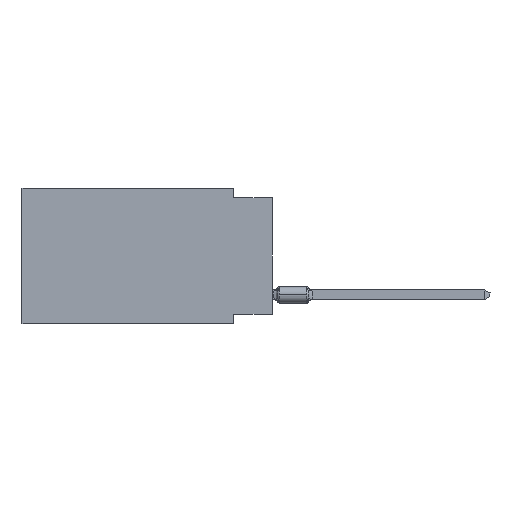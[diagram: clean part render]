
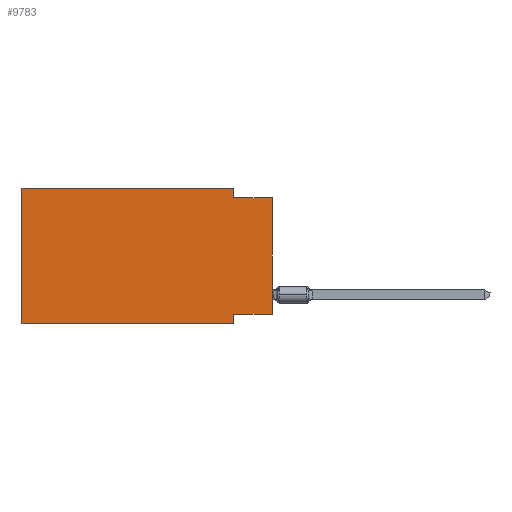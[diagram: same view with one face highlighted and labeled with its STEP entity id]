
A CAD part, left-side view. The second image highlights one B-rep face of the part: STEP entity #9783.
In plain terms, the highlighted planar face has unit normal (-1, 0, 0).
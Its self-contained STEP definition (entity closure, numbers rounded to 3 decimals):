
#138 = VERTEX_POINT ( 'NONE', #35440 ) ;
#205 = CARTESIAN_POINT ( 'NONE',  ( 0., 16.383, 0. ) ) ;
#745 = ORIENTED_EDGE ( 'NONE', *, *, #3948, .F. ) ;
#858 = DIRECTION ( 'NONE',  ( 1., 0., 0. ) ) ;
#873 = LINE ( 'NONE', #11463, #5144 ) ;
#1146 = EDGE_CURVE ( 'NONE', #31662, #40029, #20476, .T. ) ;
#1356 = VERTEX_POINT ( 'NONE', #39842 ) ;
#1871 = VERTEX_POINT ( 'NONE', #23699 ) ;
#2549 = LINE ( 'NONE', #33441, #22198 ) ;
#2625 = CARTESIAN_POINT ( 'NONE',  ( 0., 2.54, -8.89 ) ) ;
#3072 = LINE ( 'NONE', #205, #10060 ) ;
#3726 = FACE_OUTER_BOUND ( 'NONE', #29247, .T. ) ;
#3946 = CARTESIAN_POINT ( 'NONE',  ( 0., 16.383, 0. ) ) ;
#3948 = EDGE_CURVE ( 'NONE', #138, #4525, #3072, .T. ) ;
#4525 = VERTEX_POINT ( 'NONE', #18539 ) ;
#5144 = VECTOR ( 'NONE', #38138, 1000. ) ;
#5912 = LINE ( 'NONE', #2625, #37120 ) ;
#6552 = CARTESIAN_POINT ( 'NONE',  ( 0., 16.383, -8.89 ) ) ;
#6818 = DIRECTION ( 'NONE',  ( 0., 0., -1. ) ) ;
#7232 = VECTOR ( 'NONE', #14367, 1000. ) ;
#7690 = CARTESIAN_POINT ( 'NONE',  ( 0., 0., -8.255 ) ) ;
#9783 = ADVANCED_FACE ( 'NONE', ( #3726 ), #27144, .F. ) ;
#9858 = ORIENTED_EDGE ( 'NONE', *, *, #39372, .T. ) ;
#10060 = VECTOR ( 'NONE', #10582, 1000. ) ;
#10582 = DIRECTION ( 'NONE',  ( 0., 0., 1. ) ) ;
#11132 = CARTESIAN_POINT ( 'NONE',  ( 0., 2.54, -8.89 ) ) ;
#11463 = CARTESIAN_POINT ( 'NONE',  ( 0., 0., 0. ) ) ;
#12871 = DIRECTION ( 'NONE',  ( 0., -1., 0. ) ) ;
#13057 = EDGE_CURVE ( 'NONE', #1871, #35062, #5912, .T. ) ;
#13925 = ORIENTED_EDGE ( 'NONE', *, *, #23157, .F. ) ;
#14367 = DIRECTION ( 'NONE',  ( 0., 1., 0. ) ) ;
#14634 = ORIENTED_EDGE ( 'NONE', *, *, #30219, .F. ) ;
#15038 = DIRECTION ( 'NONE',  ( 0., -1., 0. ) ) ;
#15153 = EDGE_CURVE ( 'NONE', #4525, #31662, #2549, .T. ) ;
#15992 = ORIENTED_EDGE ( 'NONE', *, *, #13057, .F. ) ;
#18539 = CARTESIAN_POINT ( 'NONE',  ( 0., 16.383, 0. ) ) ;
#19082 = VERTEX_POINT ( 'NONE', #7690 ) ;
#20476 = LINE ( 'NONE', #24014, #36927 ) ;
#20486 = DIRECTION ( 'NONE',  ( 0., 0., -1. ) ) ;
#21554 = LINE ( 'NONE', #38530, #35838 ) ;
#22133 = ORIENTED_EDGE ( 'NONE', *, *, #36055, .T. ) ;
#22198 = VECTOR ( 'NONE', #36741, 1000. ) ;
#22958 = VECTOR ( 'NONE', #15038, 1000. ) ;
#23157 = EDGE_CURVE ( 'NONE', #19082, #1871, #36664, .T. ) ;
#23699 = CARTESIAN_POINT ( 'NONE',  ( 0., 2.54, -8.255 ) ) ;
#24014 = CARTESIAN_POINT ( 'NONE',  ( 0., 2.54, 0. ) ) ;
#25016 = ORIENTED_EDGE ( 'NONE', *, *, #15153, .F. ) ;
#26099 = CARTESIAN_POINT ( 'NONE',  ( 0., 0., -8.255 ) ) ;
#26667 = LINE ( 'NONE', #6552, #22958 ) ;
#27144 = PLANE ( 'NONE',  #39819 ) ;
#29247 = EDGE_LOOP ( 'NONE', ( #22133, #14634, #31177, #25016, #745, #9858, #15992, #13925 ) ) ;
#30219 = EDGE_CURVE ( 'NONE', #40029, #1356, #21554, .T. ) ;
#31058 = DIRECTION ( 'NONE',  ( 0., 0., -1. ) ) ;
#31177 = ORIENTED_EDGE ( 'NONE', *, *, #1146, .F. ) ;
#31662 = VERTEX_POINT ( 'NONE', #36081 ) ;
#33441 = CARTESIAN_POINT ( 'NONE',  ( 0., 16.383, 0. ) ) ;
#35062 = VERTEX_POINT ( 'NONE', #11132 ) ;
#35440 = CARTESIAN_POINT ( 'NONE',  ( 0., 16.383, -8.89 ) ) ;
#35838 = VECTOR ( 'NONE', #12871, 1000. ) ;
#36055 = EDGE_CURVE ( 'NONE', #19082, #1356, #873, .T. ) ;
#36081 = CARTESIAN_POINT ( 'NONE',  ( 0., 2.54, 0. ) ) ;
#36664 = LINE ( 'NONE', #26099, #7232 ) ;
#36741 = DIRECTION ( 'NONE',  ( 0., -1., 0. ) ) ;
#36927 = VECTOR ( 'NONE', #31058, 1000. ) ;
#37120 = VECTOR ( 'NONE', #20486, 1000. ) ;
#38041 = CARTESIAN_POINT ( 'NONE',  ( 0., 2.54, -0.635 ) ) ;
#38138 = DIRECTION ( 'NONE',  ( 0., 0., 1. ) ) ;
#38530 = CARTESIAN_POINT ( 'NONE',  ( 0., 0., -0.635 ) ) ;
#39372 = EDGE_CURVE ( 'NONE', #138, #35062, #26667, .T. ) ;
#39819 = AXIS2_PLACEMENT_3D ( 'NONE', #3946, #858, #6818 ) ;
#39842 = CARTESIAN_POINT ( 'NONE',  ( 0., 0., -0.635 ) ) ;
#40029 = VERTEX_POINT ( 'NONE', #38041 ) ;
